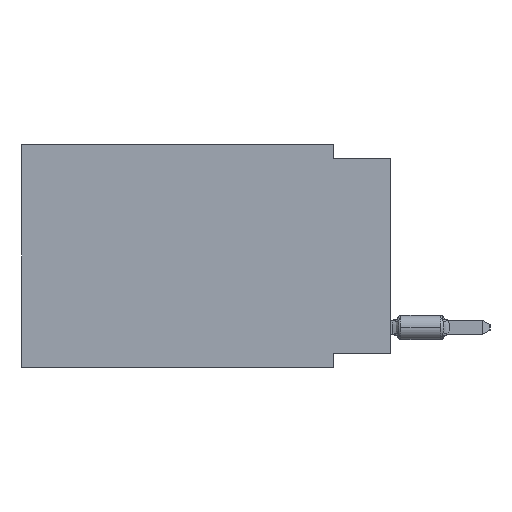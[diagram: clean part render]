
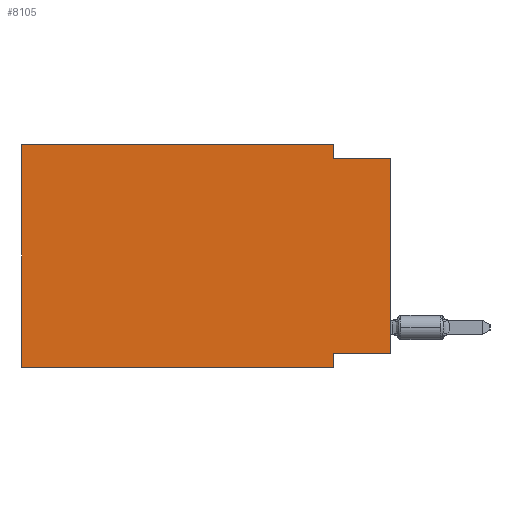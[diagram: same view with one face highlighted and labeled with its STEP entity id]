
A CAD part, left-side view. The second image highlights one B-rep face of the part: STEP entity #8105.
In plain terms, the highlighted planar face has unit normal (-1, 0, 0).
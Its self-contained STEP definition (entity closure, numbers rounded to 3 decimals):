
#407 = VERTEX_POINT ( 'NONE', #862 ) ;
#410 = CARTESIAN_POINT ( 'NONE',  ( 0., 2.54, -9.271 ) ) ;
#781 = DIRECTION ( 'NONE',  ( 0., 0., 1. ) ) ;
#862 = CARTESIAN_POINT ( 'NONE',  ( 0., 16.383, 0. ) ) ;
#1492 = DIRECTION ( 'NONE',  ( 0., 0., 1. ) ) ;
#2853 = CARTESIAN_POINT ( 'NONE',  ( 0., 0., -0.635 ) ) ;
#2989 = VERTEX_POINT ( 'NONE', #19053 ) ;
#2994 = ORIENTED_EDGE ( 'NONE', *, *, #36568, .T. ) ;
#4241 = CARTESIAN_POINT ( 'NONE',  ( 0., 0., 0. ) ) ;
#4624 = PLANE ( 'NONE',  #36865 ) ;
#5067 = DIRECTION ( 'NONE',  ( 0., 0., -1. ) ) ;
#5234 = DIRECTION ( 'NONE',  ( 0., -1., 0. ) ) ;
#5242 = VECTOR ( 'NONE', #1492, 1000. ) ;
#5394 = CARTESIAN_POINT ( 'NONE',  ( 0., 0., -9.271 ) ) ;
#5423 = DIRECTION ( 'NONE',  ( 0., 0., -1. ) ) ;
#6107 = VERTEX_POINT ( 'NONE', #19113 ) ;
#8105 = ADVANCED_FACE ( 'NONE', ( #38281 ), #4624, .F. ) ;
#8284 = EDGE_LOOP ( 'NONE', ( #2994, #33164, #10155, #22205, #26355, #10508, #37037, #40875 ) ) ;
#10155 = ORIENTED_EDGE ( 'NONE', *, *, #34177, .F. ) ;
#10392 = VECTOR ( 'NONE', #31725, 1000. ) ;
#10508 = ORIENTED_EDGE ( 'NONE', *, *, #18839, .T. ) ;
#11464 = VECTOR ( 'NONE', #5423, 1000. ) ;
#12390 = LINE ( 'NONE', #2853, #27232 ) ;
#12757 = EDGE_CURVE ( 'NONE', #14773, #6107, #25188, .T. ) ;
#13046 = EDGE_CURVE ( 'NONE', #2989, #407, #14936, .T. ) ;
#13552 = CARTESIAN_POINT ( 'NONE',  ( 0., 16.383, 0. ) ) ;
#13735 = DIRECTION ( 'NONE',  ( 0., 1., 0. ) ) ;
#14773 = VERTEX_POINT ( 'NONE', #410 ) ;
#14936 = LINE ( 'NONE', #28629, #5242 ) ;
#16601 = CARTESIAN_POINT ( 'NONE',  ( 0., 2.54, -0.635 ) ) ;
#17837 = LINE ( 'NONE', #33949, #24169 ) ;
#18839 = EDGE_CURVE ( 'NONE', #2989, #6107, #29147, .T. ) ;
#19053 = CARTESIAN_POINT ( 'NONE',  ( 0., 16.383, -9.906 ) ) ;
#19086 = CARTESIAN_POINT ( 'NONE',  ( 0., 2.54, -9.906 ) ) ;
#19113 = CARTESIAN_POINT ( 'NONE',  ( 0., 2.54, -9.906 ) ) ;
#20760 = CARTESIAN_POINT ( 'NONE',  ( 0., 2.54, 0. ) ) ;
#22205 = ORIENTED_EDGE ( 'NONE', *, *, #32750, .F. ) ;
#24169 = VECTOR ( 'NONE', #13735, 1000. ) ;
#24473 = VERTEX_POINT ( 'NONE', #5394 ) ;
#25188 = LINE ( 'NONE', #19086, #11464 ) ;
#25465 = CARTESIAN_POINT ( 'NONE',  ( 0., 16.383, 0. ) ) ;
#26355 = ORIENTED_EDGE ( 'NONE', *, *, #13046, .F. ) ;
#27232 = VECTOR ( 'NONE', #5234, 1000. ) ;
#27438 = EDGE_CURVE ( 'NONE', #32729, #42745, #12390, .T. ) ;
#28040 = LINE ( 'NONE', #38233, #10392 ) ;
#28629 = CARTESIAN_POINT ( 'NONE',  ( 0., 16.383, 0. ) ) ;
#29147 = LINE ( 'NONE', #38901, #40354 ) ;
#30083 = DIRECTION ( 'NONE',  ( 0., -1., 0. ) ) ;
#30510 = LINE ( 'NONE', #13552, #42875 ) ;
#31725 = DIRECTION ( 'NONE',  ( 0., 0., -1. ) ) ;
#32729 = VERTEX_POINT ( 'NONE', #16601 ) ;
#32750 = EDGE_CURVE ( 'NONE', #407, #33082, #30510, .T. ) ;
#33082 = VERTEX_POINT ( 'NONE', #20760 ) ;
#33164 = ORIENTED_EDGE ( 'NONE', *, *, #27438, .F. ) ;
#33949 = CARTESIAN_POINT ( 'NONE',  ( 0., 0., -9.271 ) ) ;
#34003 = LINE ( 'NONE', #4241, #38693 ) ;
#34177 = EDGE_CURVE ( 'NONE', #33082, #32729, #28040, .T. ) ;
#35107 = CARTESIAN_POINT ( 'NONE',  ( 0., 0., -0.635 ) ) ;
#36568 = EDGE_CURVE ( 'NONE', #24473, #42745, #34003, .T. ) ;
#36865 = AXIS2_PLACEMENT_3D ( 'NONE', #25465, #41520, #5067 ) ;
#36905 = EDGE_CURVE ( 'NONE', #24473, #14773, #17837, .T. ) ;
#37037 = ORIENTED_EDGE ( 'NONE', *, *, #12757, .F. ) ;
#38233 = CARTESIAN_POINT ( 'NONE',  ( 0., 2.54, 0. ) ) ;
#38281 = FACE_OUTER_BOUND ( 'NONE', #8284, .T. ) ;
#38693 = VECTOR ( 'NONE', #781, 1000. ) ;
#38901 = CARTESIAN_POINT ( 'NONE',  ( 0., 16.383, -9.906 ) ) ;
#40354 = VECTOR ( 'NONE', #42144, 1000. ) ;
#40875 = ORIENTED_EDGE ( 'NONE', *, *, #36905, .F. ) ;
#41520 = DIRECTION ( 'NONE',  ( 1., 0., 0. ) ) ;
#42144 = DIRECTION ( 'NONE',  ( 0., -1., 0. ) ) ;
#42745 = VERTEX_POINT ( 'NONE', #35107 ) ;
#42875 = VECTOR ( 'NONE', #30083, 1000. ) ;
